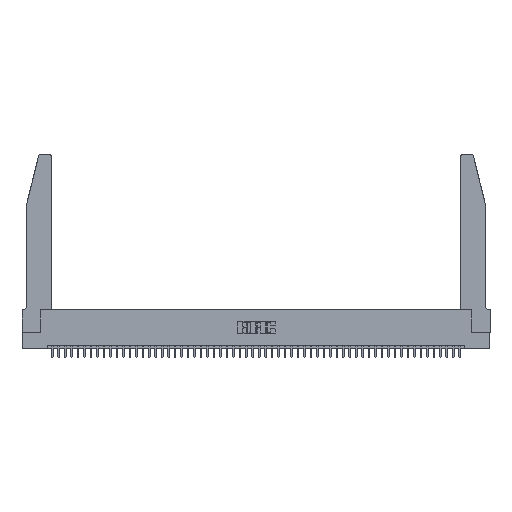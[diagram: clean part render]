
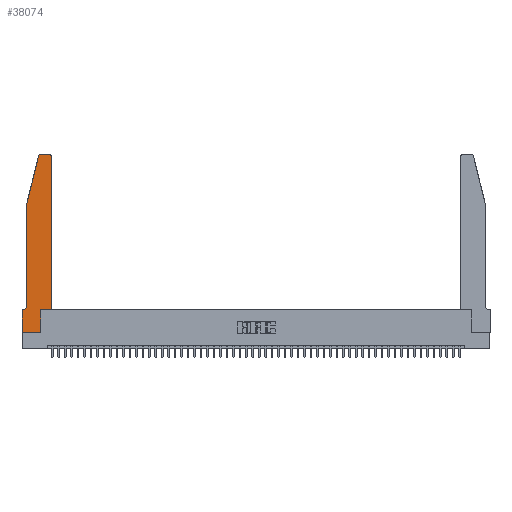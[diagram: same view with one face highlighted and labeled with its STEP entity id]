
A CAD part, top view. The second image highlights one B-rep face of the part: STEP entity #38074.
In plain terms, the highlighted planar face has unit normal (0, 0, 1).
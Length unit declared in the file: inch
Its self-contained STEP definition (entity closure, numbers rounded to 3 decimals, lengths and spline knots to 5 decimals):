
#311 = CARTESIAN_POINT ( 'NONE',  ( 0.4205, 2.72, 0.37 ) ) ;
#328 = EDGE_CURVE ( 'NONE', #41503, #22930, #28918, .T. ) ;
#634 = DIRECTION ( 'NONE',  ( 0., 0., -1. ) ) ;
#2337 = EDGE_CURVE ( 'NONE', #14350, #41503, #50544, .T. ) ;
#2489 = ORIENTED_EDGE ( 'NONE', *, *, #18806, .T. ) ;
#2657 = CARTESIAN_POINT ( 'NONE',  ( 0.4505, 2.72, 0.37 ) ) ;
#3650 = LINE ( 'NONE', #33794, #45186 ) ;
#3830 = AXIS2_PLACEMENT_3D ( 'NONE', #24875, #634, #28903 ) ;
#4315 = DIRECTION ( 'NONE',  ( 1., 0., 0. ) ) ;
#4403 = LINE ( 'NONE', #16965, #5686 ) ;
#4469 = ORIENTED_EDGE ( 'NONE', *, *, #20845, .T. ) ;
#5091 = ORIENTED_EDGE ( 'NONE', *, *, #28823, .T. ) ;
#5137 = CARTESIAN_POINT ( 'NONE',  ( 0.2865, 0.35, 0.37 ) ) ;
#5210 = LINE ( 'NONE', #51402, #34905 ) ;
#5268 = LINE ( 'NONE', #43625, #23039 ) ;
#5647 = ORIENTED_EDGE ( 'NONE', *, *, #37557, .T. ) ;
#5686 = VECTOR ( 'NONE', #44817, 39.37008 ) ;
#6560 = AXIS2_PLACEMENT_3D ( 'NONE', #43235, #19234, #47199 ) ;
#7317 = ORIENTED_EDGE ( 'NONE', *, *, #25192, .T. ) ;
#7483 = AXIS2_PLACEMENT_3D ( 'NONE', #311, #28590, #4315 ) ;
#7565 = CARTESIAN_POINT ( 'NONE',  ( 0.4505, 0.35, 0.37 ) ) ;
#9093 = VECTOR ( 'NONE', #13712, 39.37008 ) ;
#9444 = VERTEX_POINT ( 'NONE', #2657 ) ;
#9841 = CARTESIAN_POINT ( 'NONE',  ( 0.2865, 0., 0.37 ) ) ;
#9930 = ORIENTED_EDGE ( 'NONE', *, *, #18960, .T. ) ;
#13712 = DIRECTION ( 'NONE',  ( -0.239, -0.971, 0. ) ) ;
#13765 = ORIENTED_EDGE ( 'NONE', *, *, #31018, .T. ) ;
#14350 = VERTEX_POINT ( 'NONE', #45868 ) ;
#15045 = EDGE_CURVE ( 'NONE', #31251, #25937, #36079, .T. ) ;
#15348 = PLANE ( 'NONE',  #37500 ) ;
#15625 = CARTESIAN_POINT ( 'NONE',  ( 0.0055, 0.35, 0.37 ) ) ;
#15693 = ORIENTED_EDGE ( 'NONE', *, *, #36166, .T. ) ;
#16965 = CARTESIAN_POINT ( 'NONE',  ( 0., 0., 0.37 ) ) ;
#16988 = DIRECTION ( 'NONE',  ( 0., -1., 0. ) ) ;
#17479 = ORIENTED_EDGE ( 'NONE', *, *, #328, .T. ) ;
#17517 = LINE ( 'NONE', #24761, #26968 ) ;
#17578 = VERTEX_POINT ( 'NONE', #34437 ) ;
#17622 = ORIENTED_EDGE ( 'NONE', *, *, #2337, .T. ) ;
#18523 = DIRECTION ( 'NONE',  ( -1., 0., 0. ) ) ;
#18806 = EDGE_CURVE ( 'NONE', #19220, #50462, #5268, .T. ) ;
#18960 = EDGE_CURVE ( 'NONE', #9444, #31251, #29943, .T. ) ;
#19220 = VERTEX_POINT ( 'NONE', #9841 ) ;
#19234 = DIRECTION ( 'NONE',  ( 0., 0., 1. ) ) ;
#19417 = DIRECTION ( 'NONE',  ( 0., 1., 0. ) ) ;
#19430 = DIRECTION ( 'NONE',  ( 1., 0., 0. ) ) ;
#19791 = VECTOR ( 'NONE', #23513, 39.37008 ) ;
#20619 = VERTEX_POINT ( 'NONE', #7565 ) ;
#20845 = EDGE_CURVE ( 'NONE', #17578, #19220, #4403, .T. ) ;
#21609 = EDGE_CURVE ( 'NONE', #25937, #29235, #41556, .T. ) ;
#22930 = VERTEX_POINT ( 'NONE', #46908 ) ;
#23039 = VECTOR ( 'NONE', #51446, 39.37008 ) ;
#23513 = DIRECTION ( 'NONE',  ( 1., 0., 0. ) ) ;
#24761 = CARTESIAN_POINT ( 'NONE',  ( 0., 0., 0.37 ) ) ;
#24875 = CARTESIAN_POINT ( 'NONE',  ( 0.0055, 0.42, 0.37 ) ) ;
#25192 = EDGE_CURVE ( 'NONE', #39927, #14350, #3650, .T. ) ;
#25937 = VERTEX_POINT ( 'NONE', #34072 ) ;
#26968 = VECTOR ( 'NONE', #16988, 39.37008 ) ;
#28590 = DIRECTION ( 'NONE',  ( 0., 0., 1. ) ) ;
#28823 = EDGE_CURVE ( 'NONE', #20619, #9444, #5210, .T. ) ;
#28903 = DIRECTION ( 'NONE',  ( -1., 0., 0. ) ) ;
#28918 = LINE ( 'NONE', #31505, #48884 ) ;
#29235 = VERTEX_POINT ( 'NONE', #42319 ) ;
#29743 = CARTESIAN_POINT ( 'NONE',  ( 0.0755, 2., 0.37 ) ) ;
#29765 = ORIENTED_EDGE ( 'NONE', *, *, #15045, .T. ) ;
#29877 = FACE_OUTER_BOUND ( 'NONE', #33307, .T. ) ;
#29943 = CIRCLE ( 'NONE', #7483, 0.03 ) ;
#30482 = LINE ( 'NONE', #39459, #19791 ) ;
#30564 = LINE ( 'NONE', #29743, #9093 ) ;
#31018 = EDGE_CURVE ( 'NONE', #29235, #39927, #30564, .T. ) ;
#31251 = VERTEX_POINT ( 'NONE', #47151 ) ;
#31505 = CARTESIAN_POINT ( 'NONE',  ( 0.0755, 0.35, 0.37 ) ) ;
#32118 = ORIENTED_EDGE ( 'NONE', *, *, #21609, .T. ) ;
#33307 = EDGE_LOOP ( 'NONE', ( #29765, #32118, #13765, #7317, #17622, #17479, #15693, #4469, #2489, #5647, #5091, #9930 ) ) ;
#33794 = CARTESIAN_POINT ( 'NONE',  ( 0.0755, 2., 0.37 ) ) ;
#34072 = CARTESIAN_POINT ( 'NONE',  ( 0.284, 2.75, 0.37 ) ) ;
#34437 = CARTESIAN_POINT ( 'NONE',  ( 0., 0., 0.37 ) ) ;
#34905 = VECTOR ( 'NONE', #19417, 39.37008 ) ;
#35517 = DIRECTION ( 'NONE',  ( -1., 0., 0. ) ) ;
#36079 = LINE ( 'NONE', #38516, #45417 ) ;
#36166 = EDGE_CURVE ( 'NONE', #22930, #17578, #17517, .T. ) ;
#37500 = AXIS2_PLACEMENT_3D ( 'NONE', #39416, #43427, #19430 ) ;
#37557 = EDGE_CURVE ( 'NONE', #50462, #20619, #30482, .T. ) ;
#37813 = DIRECTION ( 'NONE',  ( 0., -1., 0. ) ) ;
#38074 = ADVANCED_FACE ( 'NONE', ( #29877 ), #15348, .T. ) ;
#38516 = CARTESIAN_POINT ( 'NONE',  ( 0.2605, 2.75, 0.37 ) ) ;
#39416 = CARTESIAN_POINT ( 'NONE',  ( 0., 0.35, 0.37 ) ) ;
#39459 = CARTESIAN_POINT ( 'NONE',  ( 0.4505, 0.35, 0.37 ) ) ;
#39927 = VERTEX_POINT ( 'NONE', #49387 ) ;
#41503 = VERTEX_POINT ( 'NONE', #15625 ) ;
#41556 = CIRCLE ( 'NONE', #6560, 0.03 ) ;
#42319 = CARTESIAN_POINT ( 'NONE',  ( 0.25487, 2.72718, 0.37 ) ) ;
#43235 = CARTESIAN_POINT ( 'NONE',  ( 0.284, 2.72, 0.37 ) ) ;
#43427 = DIRECTION ( 'NONE',  ( 0., 0., 1. ) ) ;
#43625 = CARTESIAN_POINT ( 'NONE',  ( 0.2865, 0.35, 0.37 ) ) ;
#44817 = DIRECTION ( 'NONE',  ( 1., 0., 0. ) ) ;
#45186 = VECTOR ( 'NONE', #37813, 39.37008 ) ;
#45417 = VECTOR ( 'NONE', #18523, 39.37008 ) ;
#45868 = CARTESIAN_POINT ( 'NONE',  ( 0.0755, 0.42, 0.37 ) ) ;
#46908 = CARTESIAN_POINT ( 'NONE',  ( 0., 0.35, 0.37 ) ) ;
#47151 = CARTESIAN_POINT ( 'NONE',  ( 0.4205, 2.75, 0.37 ) ) ;
#47199 = DIRECTION ( 'NONE',  ( 1., 0., 0. ) ) ;
#48884 = VECTOR ( 'NONE', #35517, 39.37008 ) ;
#49387 = CARTESIAN_POINT ( 'NONE',  ( 0.0755, 2., 0.37 ) ) ;
#50462 = VERTEX_POINT ( 'NONE', #5137 ) ;
#50544 = CIRCLE ( 'NONE', #3830, 0.07 ) ;
#51402 = CARTESIAN_POINT ( 'NONE',  ( 0.4505, 0.35, 0.37 ) ) ;
#51446 = DIRECTION ( 'NONE',  ( 0., 1., 0. ) ) ;
